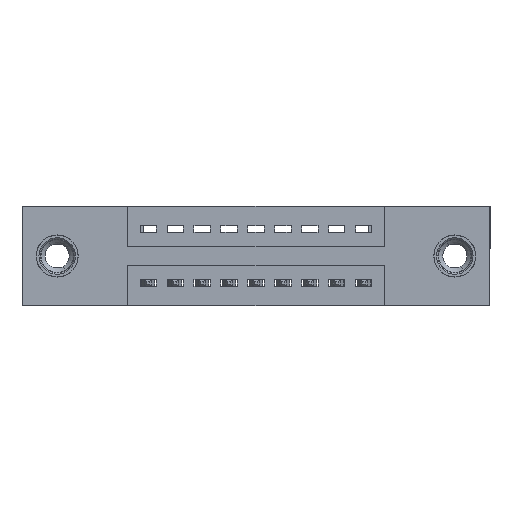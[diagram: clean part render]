
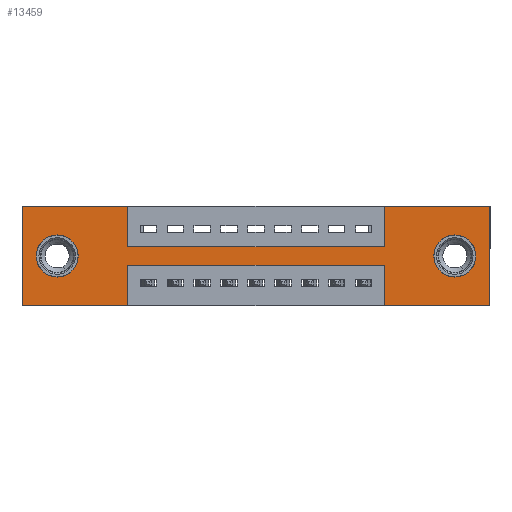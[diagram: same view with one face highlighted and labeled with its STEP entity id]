
A CAD part, front view. The second image highlights one B-rep face of the part: STEP entity #13459.
In plain terms, the highlighted planar face has unit normal (0, -1, 0).
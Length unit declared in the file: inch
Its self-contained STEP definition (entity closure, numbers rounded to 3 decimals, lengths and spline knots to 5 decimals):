
#52 = VERTEX_POINT ( 'NONE', #4784 ) ;
#131 = VERTEX_POINT ( 'NONE', #1652 ) ;
#165 = VERTEX_POINT ( 'NONE', #15209 ) ;
#170 = EDGE_CURVE ( 'NONE', #131, #4701, #3751, .T. ) ;
#321 = VECTOR ( 'NONE', #13090, 39.37008 ) ;
#402 = LINE ( 'NONE', #13432, #4814 ) ;
#534 = VECTOR ( 'NONE', #1223, 39.37008 ) ;
#640 = CARTESIAN_POINT ( 'NONE',  ( 1.3425, 0., -0.37 ) ) ;
#1020 = CARTESIAN_POINT ( 'NONE',  ( 0., 0., 0. ) ) ;
#1223 = DIRECTION ( 'NONE',  ( -1., 0., 0. ) ) ;
#1235 = AXIS2_PLACEMENT_3D ( 'NONE', #13964, #12665, #7876 ) ;
#1474 = FACE_OUTER_BOUND ( 'NONE', #7158, .T. ) ;
#1495 = CIRCLE ( 'NONE', #4671, 0.078 ) ;
#1545 = VERTEX_POINT ( 'NONE', #9770 ) ;
#1626 = CARTESIAN_POINT ( 'NONE',  ( 1.735, 0., 0. ) ) ;
#1652 = CARTESIAN_POINT ( 'NONE',  ( 1.605, 0., -0.107 ) ) ;
#1726 = DIRECTION ( 'NONE',  ( 0., -1., 0. ) ) ;
#1745 = CARTESIAN_POINT ( 'NONE',  ( 1.605, 0., -0.185 ) ) ;
#1816 = CARTESIAN_POINT ( 'NONE',  ( 0.3925, 0., -0.37 ) ) ;
#1828 = EDGE_CURVE ( 'NONE', #6496, #8618, #9320, .T. ) ;
#2035 = EDGE_CURVE ( 'NONE', #4701, #131, #3536, .T. ) ;
#2240 = LINE ( 'NONE', #9664, #534 ) ;
#2311 = VECTOR ( 'NONE', #10978, 39.37008 ) ;
#2328 = CARTESIAN_POINT ( 'NONE',  ( 0.3925, 0., 0. ) ) ;
#2581 = ORIENTED_EDGE ( 'NONE', *, *, #6317, .F. ) ;
#2648 = DIRECTION ( 'NONE',  ( 1., 0., 0. ) ) ;
#2916 = VERTEX_POINT ( 'NONE', #4692 ) ;
#2945 = ORIENTED_EDGE ( 'NONE', *, *, #13738, .F. ) ;
#2967 = CARTESIAN_POINT ( 'NONE',  ( 0.3925, 0., -0.15 ) ) ;
#3190 = VECTOR ( 'NONE', #5675, 39.37008 ) ;
#3230 = FACE_BOUND ( 'NONE', #11765, .T. ) ;
#3253 = LINE ( 'NONE', #13616, #15990 ) ;
#3269 = VERTEX_POINT ( 'NONE', #11372 ) ;
#3380 = ORIENTED_EDGE ( 'NONE', *, *, #7742, .F. ) ;
#3390 = EDGE_CURVE ( 'NONE', #8618, #13388, #10058, .T. ) ;
#3431 = FACE_BOUND ( 'NONE', #15301, .T. ) ;
#3457 = DIRECTION ( 'NONE',  ( -1., 0., 0. ) ) ;
#3536 = CIRCLE ( 'NONE', #8196, 0.078 ) ;
#3583 = CARTESIAN_POINT ( 'NONE',  ( 1.735, 0., 0. ) ) ;
#3624 = DIRECTION ( 'NONE',  ( 0., 1., 0. ) ) ;
#3662 = DIRECTION ( 'NONE',  ( 0., 0., -1. ) ) ;
#3751 = CIRCLE ( 'NONE', #1235, 0.078 ) ;
#4007 = CARTESIAN_POINT ( 'NONE',  ( 1.735, 0., -0.37 ) ) ;
#4076 = DIRECTION ( 'NONE',  ( 0., 0., -1. ) ) ;
#4211 = EDGE_CURVE ( 'NONE', #1545, #6496, #13892, .T. ) ;
#4345 = DIRECTION ( 'NONE',  ( 1., 0., 0. ) ) ;
#4561 = VECTOR ( 'NONE', #2648, 39.37008 ) ;
#4671 = AXIS2_PLACEMENT_3D ( 'NONE', #13958, #6591, #15141 ) ;
#4692 = CARTESIAN_POINT ( 'NONE',  ( 0., 0., 0. ) ) ;
#4701 = VERTEX_POINT ( 'NONE', #9548 ) ;
#4784 = CARTESIAN_POINT ( 'NONE',  ( 0., 0., -0.37 ) ) ;
#4814 = VECTOR ( 'NONE', #11991, 39.37008 ) ;
#5092 = VECTOR ( 'NONE', #9796, 39.37008 ) ;
#5240 = EDGE_CURVE ( 'NONE', #8783, #1545, #3253, .T. ) ;
#5256 = ORIENTED_EDGE ( 'NONE', *, *, #2035, .T. ) ;
#5607 = EDGE_CURVE ( 'NONE', #165, #15261, #1495, .T. ) ;
#5614 = ORIENTED_EDGE ( 'NONE', *, *, #5607, .T. ) ;
#5675 = DIRECTION ( 'NONE',  ( -1., 0., 0. ) ) ;
#5755 = ORIENTED_EDGE ( 'NONE', *, *, #15446, .F. ) ;
#5897 = ORIENTED_EDGE ( 'NONE', *, *, #6780, .T. ) ;
#5978 = ORIENTED_EDGE ( 'NONE', *, *, #6052, .F. ) ;
#6029 = VECTOR ( 'NONE', #13675, 39.37008 ) ;
#6052 = EDGE_CURVE ( 'NONE', #3269, #14358, #13827, .T. ) ;
#6317 = EDGE_CURVE ( 'NONE', #2916, #14957, #11154, .T. ) ;
#6436 = VERTEX_POINT ( 'NONE', #11318 ) ;
#6469 = LINE ( 'NONE', #13478, #14355 ) ;
#6496 = VERTEX_POINT ( 'NONE', #14460 ) ;
#6591 = DIRECTION ( 'NONE',  ( 0., 1., 0. ) ) ;
#6780 = EDGE_CURVE ( 'NONE', #15261, #165, #9572, .T. ) ;
#6927 = PLANE ( 'NONE',  #11994 ) ;
#7139 = EDGE_CURVE ( 'NONE', #52, #2916, #15366, .T. ) ;
#7158 = EDGE_LOOP ( 'NONE', ( #12152, #3380, #5978, #2945, #13115, #15981, #14651, #7865, #10833, #2581, #11415, #5755 ) ) ;
#7206 = CARTESIAN_POINT ( 'NONE',  ( 0., 0., 0. ) ) ;
#7520 = LINE ( 'NONE', #9771, #14086 ) ;
#7742 = EDGE_CURVE ( 'NONE', #14358, #6436, #12259, .T. ) ;
#7865 = ORIENTED_EDGE ( 'NONE', *, *, #5240, .F. ) ;
#7876 = DIRECTION ( 'NONE',  ( 0., 0., -1. ) ) ;
#8196 = AXIS2_PLACEMENT_3D ( 'NONE', #1745, #11481, #4076 ) ;
#8618 = VERTEX_POINT ( 'NONE', #3583 ) ;
#8783 = VERTEX_POINT ( 'NONE', #2967 ) ;
#9215 = EDGE_CURVE ( 'NONE', #14957, #8783, #6469, .T. ) ;
#9320 = LINE ( 'NONE', #14854, #6029 ) ;
#9548 = CARTESIAN_POINT ( 'NONE',  ( 1.605, 0., -0.263 ) ) ;
#9572 = CIRCLE ( 'NONE', #11018, 0.078 ) ;
#9664 = CARTESIAN_POINT ( 'NONE',  ( 0., 0., -0.37 ) ) ;
#9770 = CARTESIAN_POINT ( 'NONE',  ( 1.3425, 0., -0.15 ) ) ;
#9771 = CARTESIAN_POINT ( 'NONE',  ( 0., 0., -0.37 ) ) ;
#9796 = DIRECTION ( 'NONE',  ( 0., 0., 1. ) ) ;
#9837 = CARTESIAN_POINT ( 'NONE',  ( 1.3425, 0., 0. ) ) ;
#10058 = LINE ( 'NONE', #1626, #15851 ) ;
#10614 = CARTESIAN_POINT ( 'NONE',  ( 0.3925, 0., -0.22 ) ) ;
#10833 = ORIENTED_EDGE ( 'NONE', *, *, #9215, .F. ) ;
#10978 = DIRECTION ( 'NONE',  ( 0., 0., 1. ) ) ;
#11018 = AXIS2_PLACEMENT_3D ( 'NONE', #14826, #3624, #14924 ) ;
#11051 = CARTESIAN_POINT ( 'NONE',  ( 1.3425, 0., -0.22 ) ) ;
#11154 = LINE ( 'NONE', #1020, #4561 ) ;
#11301 = ORIENTED_EDGE ( 'NONE', *, *, #170, .T. ) ;
#11318 = CARTESIAN_POINT ( 'NONE',  ( 0.3925, 0., -0.22 ) ) ;
#11372 = CARTESIAN_POINT ( 'NONE',  ( 1.3425, 0., -0.37 ) ) ;
#11415 = ORIENTED_EDGE ( 'NONE', *, *, #7139, .F. ) ;
#11481 = DIRECTION ( 'NONE',  ( 0., 1., 0. ) ) ;
#11587 = DIRECTION ( 'NONE',  ( 0., 0., -1. ) ) ;
#11620 = EDGE_CURVE ( 'NONE', #6436, #14177, #402, .T. ) ;
#11675 = CARTESIAN_POINT ( 'NONE',  ( 0.13, 0., -0.263 ) ) ;
#11765 = EDGE_LOOP ( 'NONE', ( #11301, #5256 ) ) ;
#11991 = DIRECTION ( 'NONE',  ( 0., 0., -1. ) ) ;
#11994 = AXIS2_PLACEMENT_3D ( 'NONE', #15548, #1726, #13012 ) ;
#12152 = ORIENTED_EDGE ( 'NONE', *, *, #11620, .F. ) ;
#12259 = LINE ( 'NONE', #10614, #3190 ) ;
#12665 = DIRECTION ( 'NONE',  ( 0., 1., 0. ) ) ;
#13012 = DIRECTION ( 'NONE',  ( 0., 0., -1. ) ) ;
#13090 = DIRECTION ( 'NONE',  ( 0., 0., 1. ) ) ;
#13115 = ORIENTED_EDGE ( 'NONE', *, *, #3390, .F. ) ;
#13388 = VERTEX_POINT ( 'NONE', #4007 ) ;
#13432 = CARTESIAN_POINT ( 'NONE',  ( 0.3925, 0., -0.37 ) ) ;
#13459 = ADVANCED_FACE ( 'NONE', ( #3230, #3431, #1474 ), #6927, .T. ) ;
#13478 = CARTESIAN_POINT ( 'NONE',  ( 0.3925, 0., 0. ) ) ;
#13616 = CARTESIAN_POINT ( 'NONE',  ( 0.3925, 0., -0.15 ) ) ;
#13675 = DIRECTION ( 'NONE',  ( 1., 0., 0. ) ) ;
#13738 = EDGE_CURVE ( 'NONE', #13388, #3269, #2240, .T. ) ;
#13827 = LINE ( 'NONE', #640, #321 ) ;
#13892 = LINE ( 'NONE', #9837, #2311 ) ;
#13958 = CARTESIAN_POINT ( 'NONE',  ( 0.13, 0., -0.185 ) ) ;
#13964 = CARTESIAN_POINT ( 'NONE',  ( 1.605, 0., -0.185 ) ) ;
#14086 = VECTOR ( 'NONE', #3457, 39.37008 ) ;
#14177 = VERTEX_POINT ( 'NONE', #1816 ) ;
#14355 = VECTOR ( 'NONE', #3662, 39.37008 ) ;
#14358 = VERTEX_POINT ( 'NONE', #11051 ) ;
#14460 = CARTESIAN_POINT ( 'NONE',  ( 1.3425, 0., 0. ) ) ;
#14651 = ORIENTED_EDGE ( 'NONE', *, *, #4211, .F. ) ;
#14826 = CARTESIAN_POINT ( 'NONE',  ( 0.13, 0., -0.185 ) ) ;
#14854 = CARTESIAN_POINT ( 'NONE',  ( 0., 0., 0. ) ) ;
#14924 = DIRECTION ( 'NONE',  ( 0., 0., 1. ) ) ;
#14957 = VERTEX_POINT ( 'NONE', #2328 ) ;
#15141 = DIRECTION ( 'NONE',  ( 0., 0., 1. ) ) ;
#15209 = CARTESIAN_POINT ( 'NONE',  ( 0.13, 0., -0.107 ) ) ;
#15261 = VERTEX_POINT ( 'NONE', #11675 ) ;
#15301 = EDGE_LOOP ( 'NONE', ( #5614, #5897 ) ) ;
#15366 = LINE ( 'NONE', #7206, #5092 ) ;
#15446 = EDGE_CURVE ( 'NONE', #14177, #52, #7520, .T. ) ;
#15548 = CARTESIAN_POINT ( 'NONE',  ( 0., 0., -0.37 ) ) ;
#15851 = VECTOR ( 'NONE', #11587, 39.37008 ) ;
#15981 = ORIENTED_EDGE ( 'NONE', *, *, #1828, .F. ) ;
#15990 = VECTOR ( 'NONE', #4345, 39.37008 ) ;
